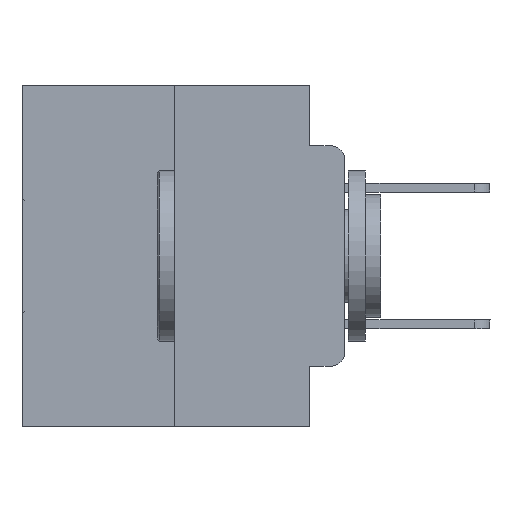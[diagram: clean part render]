
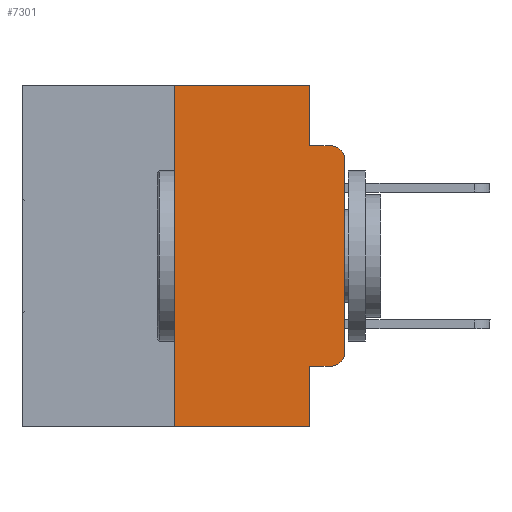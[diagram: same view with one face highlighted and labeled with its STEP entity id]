
A CAD part, left-side view. The second image highlights one B-rep face of the part: STEP entity #7301.
In plain terms, the highlighted planar face has unit normal (-1, 0, 0).
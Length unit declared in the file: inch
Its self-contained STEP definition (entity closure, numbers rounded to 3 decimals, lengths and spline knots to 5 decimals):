
#68 = LINE ( 'NONE', #4746, #8147 ) ;
#160 = DIRECTION ( 'NONE',  ( 0., 0., -1. ) ) ;
#508 = EDGE_CURVE ( 'NONE', #1924, #17688, #19978, .T. ) ;
#521 = ORIENTED_EDGE ( 'NONE', *, *, #624, .T. ) ;
#624 = EDGE_CURVE ( 'NONE', #9966, #15187, #12625, .T. ) ;
#739 = VECTOR ( 'NONE', #160, 39.37008 ) ;
#822 = DIRECTION ( 'NONE',  ( 0., 0., -1. ) ) ;
#1511 = ORIENTED_EDGE ( 'NONE', *, *, #508, .T. ) ;
#1650 = CARTESIAN_POINT ( 'NONE',  ( 0., 0.25, 0. ) ) ;
#1652 = FACE_OUTER_BOUND ( 'NONE', #22923, .T. ) ;
#1924 = VERTEX_POINT ( 'NONE', #26965 ) ;
#2192 = DIRECTION ( 'NONE',  ( 0., -1., 0. ) ) ;
#2273 = VECTOR ( 'NONE', #16891, 39.37008 ) ;
#2334 = CARTESIAN_POINT ( 'NONE',  ( 0., 0.051, -0.0885 ) ) ;
#3100 = EDGE_CURVE ( 'NONE', #4547, #9966, #7291, .T. ) ;
#3232 = VERTEX_POINT ( 'NONE', #24801 ) ;
#3307 = EDGE_CURVE ( 'NONE', #15187, #3232, #23788, .T. ) ;
#3332 = AXIS2_PLACEMENT_3D ( 'NONE', #5178, #28993, #822 ) ;
#4477 = DIRECTION ( 'NONE',  ( 0., -1., 0. ) ) ;
#4547 = VERTEX_POINT ( 'NONE', #28068 ) ;
#4746 = CARTESIAN_POINT ( 'NONE',  ( 0., 0.25, 0. ) ) ;
#5178 = CARTESIAN_POINT ( 'NONE',  ( 0., 0.02, -0.3915 ) ) ;
#6449 = CARTESIAN_POINT ( 'NONE',  ( 0., 0., -0.3915 ) ) ;
#6824 = DIRECTION ( 'NONE',  ( 0., -1., 0. ) ) ;
#6999 = LINE ( 'NONE', #16968, #11555 ) ;
#7291 = CIRCLE ( 'NONE', #3332, 0.02 ) ;
#7301 = ADVANCED_FACE ( 'NONE', ( #1652 ), #15966, .F. ) ;
#7844 = ORIENTED_EDGE ( 'NONE', *, *, #13199, .F. ) ;
#8147 = VECTOR ( 'NONE', #28714, 39.37008 ) ;
#8396 = DIRECTION ( 'NONE',  ( 0., 0., 1. ) ) ;
#8554 = ORIENTED_EDGE ( 'NONE', *, *, #22262, .T. ) ;
#8608 = AXIS2_PLACEMENT_3D ( 'NONE', #11121, #20363, #29812 ) ;
#9966 = VERTEX_POINT ( 'NONE', #6449 ) ;
#11121 = CARTESIAN_POINT ( 'NONE',  ( 0., 0.473, 0. ) ) ;
#11280 = VERTEX_POINT ( 'NONE', #1650 ) ;
#11555 = VECTOR ( 'NONE', #2192, 39.37008 ) ;
#12036 = CARTESIAN_POINT ( 'NONE',  ( 0., 0.051, 0. ) ) ;
#12047 = VECTOR ( 'NONE', #4477, 39.37008 ) ;
#12625 = LINE ( 'NONE', #29746, #30044 ) ;
#12954 = CARTESIAN_POINT ( 'NONE',  ( 0., 0.02, -0.1085 ) ) ;
#13199 = EDGE_CURVE ( 'NONE', #15170, #17688, #25925, .T. ) ;
#13264 = DIRECTION ( 'NONE',  ( 0., 0., -1. ) ) ;
#13848 = LINE ( 'NONE', #2334, #20885 ) ;
#14327 = AXIS2_PLACEMENT_3D ( 'NONE', #12954, #22471, #13264 ) ;
#14792 = LINE ( 'NONE', #28501, #739 ) ;
#15170 = VERTEX_POINT ( 'NONE', #22606 ) ;
#15187 = VERTEX_POINT ( 'NONE', #27275 ) ;
#15595 = DIRECTION ( 'NONE',  ( 0., -1., 0. ) ) ;
#15966 = PLANE ( 'NONE',  #8608 ) ;
#16062 = CARTESIAN_POINT ( 'NONE',  ( 0., 0.051, -0.0885 ) ) ;
#16198 = VERTEX_POINT ( 'NONE', #16062 ) ;
#16312 = LINE ( 'NONE', #30615, #12047 ) ;
#16891 = DIRECTION ( 'NONE',  ( 0., 0., -1. ) ) ;
#16968 = CARTESIAN_POINT ( 'NONE',  ( 0., 0.051, -0.4115 ) ) ;
#17304 = CARTESIAN_POINT ( 'NONE',  ( 0., 0.051, 0. ) ) ;
#17656 = VERTEX_POINT ( 'NONE', #17304 ) ;
#17678 = ORIENTED_EDGE ( 'NONE', *, *, #3307, .T. ) ;
#17688 = VERTEX_POINT ( 'NONE', #29423 ) ;
#19126 = ORIENTED_EDGE ( 'NONE', *, *, #21012, .F. ) ;
#19614 = VECTOR ( 'NONE', #15595, 39.37008 ) ;
#19978 = LINE ( 'NONE', #27279, #19614 ) ;
#20363 = DIRECTION ( 'NONE',  ( 1., 0., 0. ) ) ;
#20885 = VECTOR ( 'NONE', #6824, 39.37008 ) ;
#21012 = EDGE_CURVE ( 'NONE', #11280, #17656, #16312, .T. ) ;
#22262 = EDGE_CURVE ( 'NONE', #15170, #4547, #6999, .T. ) ;
#22471 = DIRECTION ( 'NONE',  ( -1., 0., 0. ) ) ;
#22606 = CARTESIAN_POINT ( 'NONE',  ( 0., 0.051, -0.4115 ) ) ;
#22923 = EDGE_LOOP ( 'NONE', ( #521, #17678, #25551, #24326, #19126, #27927, #1511, #7844, #8554, #29549 ) ) ;
#23788 = CIRCLE ( 'NONE', #14327, 0.02 ) ;
#24225 = EDGE_CURVE ( 'NONE', #1924, #11280, #68, .T. ) ;
#24326 = ORIENTED_EDGE ( 'NONE', *, *, #24828, .F. ) ;
#24801 = CARTESIAN_POINT ( 'NONE',  ( 0., 0.02, -0.0885 ) ) ;
#24828 = EDGE_CURVE ( 'NONE', #17656, #16198, #14792, .T. ) ;
#25551 = ORIENTED_EDGE ( 'NONE', *, *, #30670, .F. ) ;
#25925 = LINE ( 'NONE', #12036, #2273 ) ;
#26965 = CARTESIAN_POINT ( 'NONE',  ( 0., 0.25, -0.5 ) ) ;
#27275 = CARTESIAN_POINT ( 'NONE',  ( 0., 0., -0.1085 ) ) ;
#27279 = CARTESIAN_POINT ( 'NONE',  ( 0., 0.473, -0.5 ) ) ;
#27927 = ORIENTED_EDGE ( 'NONE', *, *, #24225, .F. ) ;
#28068 = CARTESIAN_POINT ( 'NONE',  ( 0., 0.02, -0.4115 ) ) ;
#28501 = CARTESIAN_POINT ( 'NONE',  ( 0., 0.051, 0. ) ) ;
#28714 = DIRECTION ( 'NONE',  ( 0., 0., 1. ) ) ;
#28993 = DIRECTION ( 'NONE',  ( -1., 0., 0. ) ) ;
#29423 = CARTESIAN_POINT ( 'NONE',  ( 0., 0.051, -0.5 ) ) ;
#29549 = ORIENTED_EDGE ( 'NONE', *, *, #3100, .T. ) ;
#29746 = CARTESIAN_POINT ( 'NONE',  ( 0., 0., 0. ) ) ;
#29812 = DIRECTION ( 'NONE',  ( 0., 0., -1. ) ) ;
#30044 = VECTOR ( 'NONE', #8396, 39.37008 ) ;
#30615 = CARTESIAN_POINT ( 'NONE',  ( 0., 0.473, 0. ) ) ;
#30670 = EDGE_CURVE ( 'NONE', #16198, #3232, #13848, .T. ) ;
